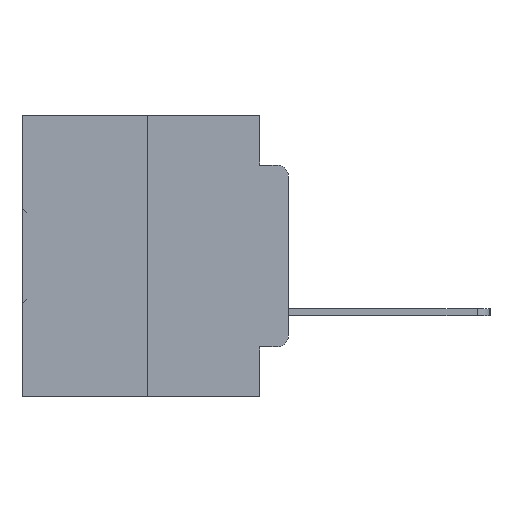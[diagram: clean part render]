
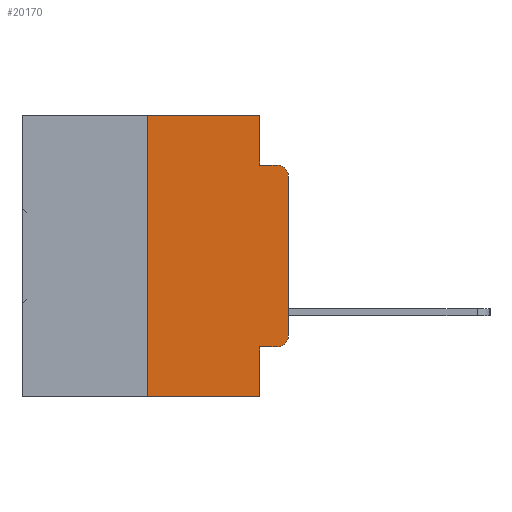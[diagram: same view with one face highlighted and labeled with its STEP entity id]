
A CAD part, left-side view. The second image highlights one B-rep face of the part: STEP entity #20170.
In plain terms, the highlighted planar face has unit normal (-1, 0, 0).
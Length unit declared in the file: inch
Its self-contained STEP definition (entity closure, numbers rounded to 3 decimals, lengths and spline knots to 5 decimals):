
#553 = DIRECTION ( 'NONE',  ( 0., 0., -1. ) ) ;
#1290 = CARTESIAN_POINT ( 'NONE',  ( 0., 0., -0.1085 ) ) ;
#2323 = CARTESIAN_POINT ( 'NONE',  ( 0., 0.02, -0.3915 ) ) ;
#2775 = EDGE_CURVE ( 'NONE', #33271, #31974, #22553, .T. ) ;
#3420 = VERTEX_POINT ( 'NONE', #34029 ) ;
#3548 = ORIENTED_EDGE ( 'NONE', *, *, #2775, .T. ) ;
#5030 = LINE ( 'NONE', #7176, #11372 ) ;
#5119 = DIRECTION ( 'NONE',  ( 0., 0., -1. ) ) ;
#5339 = ORIENTED_EDGE ( 'NONE', *, *, #14429, .F. ) ;
#5743 = DIRECTION ( 'NONE',  ( 0., -1., 0. ) ) ;
#5839 = VECTOR ( 'NONE', #5743, 39.37008 ) ;
#7176 = CARTESIAN_POINT ( 'NONE',  ( 0., 0.25, 0. ) ) ;
#7328 = VERTEX_POINT ( 'NONE', #28169 ) ;
#7434 = LINE ( 'NONE', #30363, #27965 ) ;
#7545 = LINE ( 'NONE', #19215, #5839 ) ;
#8089 = CARTESIAN_POINT ( 'NONE',  ( 0., 0.25, -0.5 ) ) ;
#8231 = VECTOR ( 'NONE', #30809, 39.37008 ) ;
#8666 = DIRECTION ( 'NONE',  ( -1., 0., 0. ) ) ;
#9277 = AXIS2_PLACEMENT_3D ( 'NONE', #19439, #16838, #553 ) ;
#9463 = CARTESIAN_POINT ( 'NONE',  ( 0., 0.051, 0. ) ) ;
#9500 = CARTESIAN_POINT ( 'NONE',  ( 0., 0.051, 0. ) ) ;
#10783 = EDGE_CURVE ( 'NONE', #3420, #33271, #24862, .T. ) ;
#11372 = VECTOR ( 'NONE', #31247, 39.37008 ) ;
#11416 = PLANE ( 'NONE',  #9277 ) ;
#11516 = VECTOR ( 'NONE', #25198, 39.37008 ) ;
#12187 = DIRECTION ( 'NONE',  ( 0., 0., -1. ) ) ;
#12579 = EDGE_CURVE ( 'NONE', #22500, #3420, #16917, .T. ) ;
#13843 = ORIENTED_EDGE ( 'NONE', *, *, #10783, .T. ) ;
#14028 = AXIS2_PLACEMENT_3D ( 'NONE', #2323, #21259, #5119 ) ;
#14154 = CARTESIAN_POINT ( 'NONE',  ( 0., 0.02, -0.0885 ) ) ;
#14429 = EDGE_CURVE ( 'NONE', #24491, #15527, #7545, .T. ) ;
#14704 = FACE_OUTER_BOUND ( 'NONE', #19463, .T. ) ;
#15361 = DIRECTION ( 'NONE',  ( 0., 0., -1. ) ) ;
#15527 = VERTEX_POINT ( 'NONE', #9500 ) ;
#15812 = CARTESIAN_POINT ( 'NONE',  ( 0., 0., -0.3915 ) ) ;
#16441 = LINE ( 'NONE', #9463, #29743 ) ;
#16751 = ORIENTED_EDGE ( 'NONE', *, *, #19813, .F. ) ;
#16838 = DIRECTION ( 'NONE',  ( 1., 0., 0. ) ) ;
#16917 = LINE ( 'NONE', #24113, #23206 ) ;
#17196 = ORIENTED_EDGE ( 'NONE', *, *, #17816, .T. ) ;
#17816 = EDGE_CURVE ( 'NONE', #34000, #24633, #32738, .T. ) ;
#18019 = EDGE_CURVE ( 'NONE', #22500, #24633, #19103, .T. ) ;
#18020 = ORIENTED_EDGE ( 'NONE', *, *, #26939, .F. ) ;
#19103 = LINE ( 'NONE', #20664, #32320 ) ;
#19215 = CARTESIAN_POINT ( 'NONE',  ( 0., 0.473, 0. ) ) ;
#19439 = CARTESIAN_POINT ( 'NONE',  ( 0., 0.473, 0. ) ) ;
#19463 = EDGE_LOOP ( 'NONE', ( #3548, #31673, #23443, #18020, #5339, #16751, #17196, #25968, #32536, #13843 ) ) ;
#19813 = EDGE_CURVE ( 'NONE', #34000, #24491, #5030, .T. ) ;
#20110 = CARTESIAN_POINT ( 'NONE',  ( 0., 0.051, -0.4115 ) ) ;
#20170 = ADVANCED_FACE ( 'NONE', ( #14704 ), #11416, .F. ) ;
#20664 = CARTESIAN_POINT ( 'NONE',  ( 0., 0.051, 0. ) ) ;
#21259 = DIRECTION ( 'NONE',  ( -1., 0., 0. ) ) ;
#22500 = VERTEX_POINT ( 'NONE', #20110 ) ;
#22538 = CARTESIAN_POINT ( 'NONE',  ( 0., 0.473, -0.5 ) ) ;
#22553 = LINE ( 'NONE', #29269, #8231 ) ;
#23206 = VECTOR ( 'NONE', #26782, 39.37008 ) ;
#23443 = ORIENTED_EDGE ( 'NONE', *, *, #28687, .F. ) ;
#23467 = CARTESIAN_POINT ( 'NONE',  ( 0., 0.051, -0.5 ) ) ;
#24113 = CARTESIAN_POINT ( 'NONE',  ( 0., 0.051, -0.4115 ) ) ;
#24491 = VERTEX_POINT ( 'NONE', #30735 ) ;
#24633 = VERTEX_POINT ( 'NONE', #23467 ) ;
#24768 = CARTESIAN_POINT ( 'NONE',  ( 0., 0.02, -0.1085 ) ) ;
#24862 = CIRCLE ( 'NONE', #14028, 0.02 ) ;
#25074 = DIRECTION ( 'NONE',  ( 0., -1., 0. ) ) ;
#25198 = DIRECTION ( 'NONE',  ( 0., -1., 0. ) ) ;
#25968 = ORIENTED_EDGE ( 'NONE', *, *, #18019, .F. ) ;
#26782 = DIRECTION ( 'NONE',  ( 0., -1., 0. ) ) ;
#26939 = EDGE_CURVE ( 'NONE', #15527, #7328, #16441, .T. ) ;
#27360 = VERTEX_POINT ( 'NONE', #14154 ) ;
#27436 = DIRECTION ( 'NONE',  ( 0., 0., -1. ) ) ;
#27692 = AXIS2_PLACEMENT_3D ( 'NONE', #24768, #8666, #27436 ) ;
#27965 = VECTOR ( 'NONE', #25074, 39.37008 ) ;
#28169 = CARTESIAN_POINT ( 'NONE',  ( 0., 0.051, -0.0885 ) ) ;
#28687 = EDGE_CURVE ( 'NONE', #7328, #27360, #7434, .T. ) ;
#29269 = CARTESIAN_POINT ( 'NONE',  ( 0., 0., 0. ) ) ;
#29743 = VECTOR ( 'NONE', #12187, 39.37008 ) ;
#29787 = CIRCLE ( 'NONE', #27692, 0.02 ) ;
#30363 = CARTESIAN_POINT ( 'NONE',  ( 0., 0.051, -0.0885 ) ) ;
#30439 = EDGE_CURVE ( 'NONE', #31974, #27360, #29787, .T. ) ;
#30735 = CARTESIAN_POINT ( 'NONE',  ( 0., 0.25, 0. ) ) ;
#30809 = DIRECTION ( 'NONE',  ( 0., 0., 1. ) ) ;
#31247 = DIRECTION ( 'NONE',  ( 0., 0., 1. ) ) ;
#31673 = ORIENTED_EDGE ( 'NONE', *, *, #30439, .T. ) ;
#31974 = VERTEX_POINT ( 'NONE', #1290 ) ;
#32320 = VECTOR ( 'NONE', #15361, 39.37008 ) ;
#32536 = ORIENTED_EDGE ( 'NONE', *, *, #12579, .T. ) ;
#32738 = LINE ( 'NONE', #22538, #11516 ) ;
#33271 = VERTEX_POINT ( 'NONE', #15812 ) ;
#34000 = VERTEX_POINT ( 'NONE', #8089 ) ;
#34029 = CARTESIAN_POINT ( 'NONE',  ( 0., 0.02, -0.4115 ) ) ;
